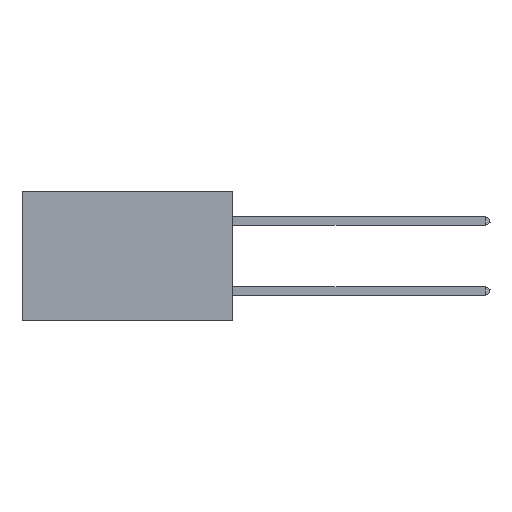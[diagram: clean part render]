
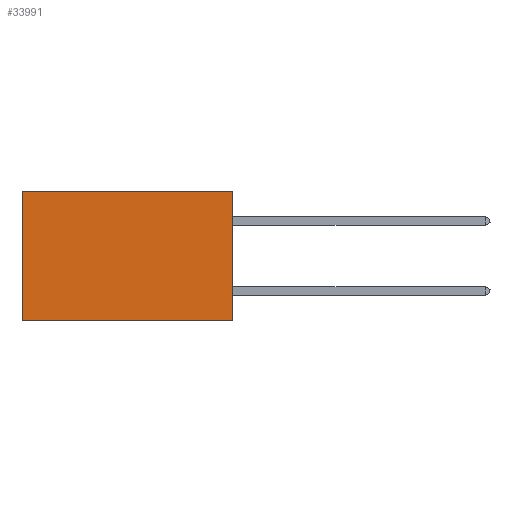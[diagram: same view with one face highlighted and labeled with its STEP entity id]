
A CAD part, left-side view. The second image highlights one B-rep face of the part: STEP entity #33991.
In plain terms, the highlighted planar face has unit normal (-1, 0, 0).
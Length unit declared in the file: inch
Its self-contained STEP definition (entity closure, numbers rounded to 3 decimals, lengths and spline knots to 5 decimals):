
#1240 = CARTESIAN_POINT ( 'NONE',  ( 0.2875, 0., -0.37 ) ) ;
#3718 = DIRECTION ( 'NONE',  ( 0., 1., 0. ) ) ;
#4075 = CARTESIAN_POINT ( 'NONE',  ( 0.2875, 0.6, 0. ) ) ;
#4653 = EDGE_LOOP ( 'NONE', ( #35748, #12444, #36061, #11383 ) ) ;
#5883 = AXIS2_PLACEMENT_3D ( 'NONE', #35407, #18811, #13559 ) ;
#6860 = EDGE_CURVE ( 'NONE', #11692, #23765, #18176, .T. ) ;
#7398 = PLANE ( 'NONE',  #5883 ) ;
#10146 = LINE ( 'NONE', #13880, #28993 ) ;
#11383 = ORIENTED_EDGE ( 'NONE', *, *, #13511, .T. ) ;
#11692 = VERTEX_POINT ( 'NONE', #16840 ) ;
#12444 = ORIENTED_EDGE ( 'NONE', *, *, #6860, .F. ) ;
#13351 = DIRECTION ( 'NONE',  ( 0., 0., -1. ) ) ;
#13511 = EDGE_CURVE ( 'NONE', #21051, #25763, #10146, .T. ) ;
#13559 = DIRECTION ( 'NONE',  ( 0., 0., -1. ) ) ;
#13880 = CARTESIAN_POINT ( 'NONE',  ( 0.2875, 0., 0. ) ) ;
#16267 = CARTESIAN_POINT ( 'NONE',  ( 0.2875, 0.6, 0. ) ) ;
#16840 = CARTESIAN_POINT ( 'NONE',  ( 0.2875, 0., -0.37 ) ) ;
#17035 = VECTOR ( 'NONE', #13351, 39.37008 ) ;
#17970 = FACE_OUTER_BOUND ( 'NONE', #4653, .T. ) ;
#18176 = LINE ( 'NONE', #1240, #34453 ) ;
#18811 = DIRECTION ( 'NONE',  ( 1., 0., 0. ) ) ;
#21051 = VERTEX_POINT ( 'NONE', #22982 ) ;
#22170 = EDGE_CURVE ( 'NONE', #21051, #11692, #31571, .T. ) ;
#22982 = CARTESIAN_POINT ( 'NONE',  ( 0.2875, 0., 0. ) ) ;
#23223 = VECTOR ( 'NONE', #31818, 39.37008 ) ;
#23765 = VERTEX_POINT ( 'NONE', #27123 ) ;
#25763 = VERTEX_POINT ( 'NONE', #4075 ) ;
#25914 = CARTESIAN_POINT ( 'NONE',  ( 0.2875, 0., 0. ) ) ;
#27123 = CARTESIAN_POINT ( 'NONE',  ( 0.2875, 0.6, -0.37 ) ) ;
#28993 = VECTOR ( 'NONE', #30306, 39.37008 ) ;
#30306 = DIRECTION ( 'NONE',  ( 0., 1., 0. ) ) ;
#31571 = LINE ( 'NONE', #25914, #23223 ) ;
#31818 = DIRECTION ( 'NONE',  ( 0., 0., -1. ) ) ;
#33991 = ADVANCED_FACE ( 'NONE', ( #17970 ), #7398, .F. ) ;
#34453 = VECTOR ( 'NONE', #3718, 39.37008 ) ;
#34585 = EDGE_CURVE ( 'NONE', #25763, #23765, #34643, .T. ) ;
#34643 = LINE ( 'NONE', #16267, #17035 ) ;
#35407 = CARTESIAN_POINT ( 'NONE',  ( 0.2875, 0., 0. ) ) ;
#35748 = ORIENTED_EDGE ( 'NONE', *, *, #34585, .T. ) ;
#36061 = ORIENTED_EDGE ( 'NONE', *, *, #22170, .F. ) ;
